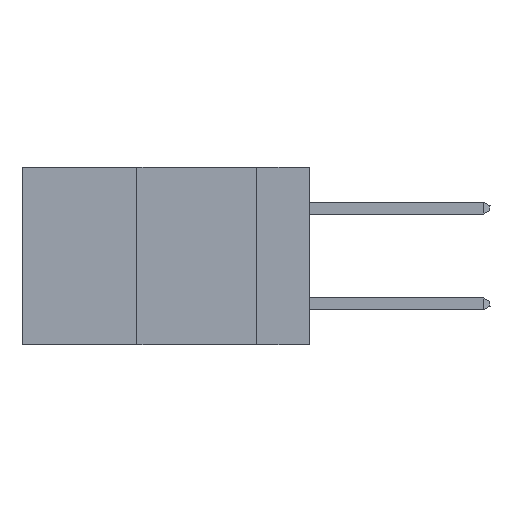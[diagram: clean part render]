
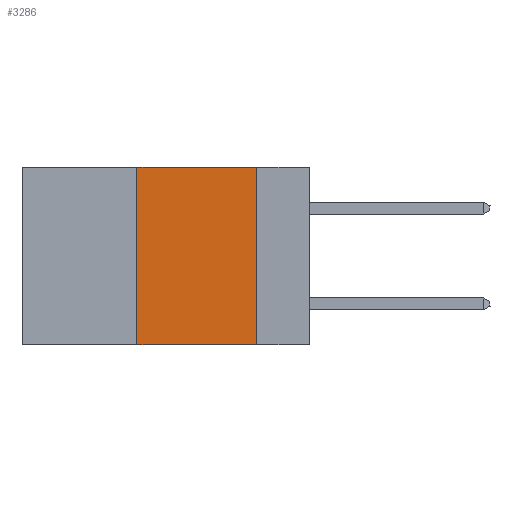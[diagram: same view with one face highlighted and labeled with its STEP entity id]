
A CAD part, left-side view. The second image highlights one B-rep face of the part: STEP entity #3286.
In plain terms, the highlighted planar face has unit normal (-1, 0, 0).
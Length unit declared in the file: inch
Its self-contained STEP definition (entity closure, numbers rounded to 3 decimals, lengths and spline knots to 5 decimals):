
#913 = ORIENTED_EDGE ( 'NONE', *, *, #22457, .F. ) ;
#1438 = CARTESIAN_POINT ( 'NONE',  ( 0., 0.11, 0. ) ) ;
#2616 = VECTOR ( 'NONE', #3526, 39.37008 ) ;
#3018 = FACE_OUTER_BOUND ( 'NONE', #5909, .T. ) ;
#3286 = ADVANCED_FACE ( 'NONE', ( #3018 ), #4682, .F. ) ;
#3526 = DIRECTION ( 'NONE',  ( 0., -1., 0. ) ) ;
#4585 = DIRECTION ( 'NONE',  ( 0., 0., -1. ) ) ;
#4609 = DIRECTION ( 'NONE',  ( 1., 0., 0. ) ) ;
#4682 = PLANE ( 'NONE',  #16794 ) ;
#5305 = CARTESIAN_POINT ( 'NONE',  ( 0., 0.6, 0. ) ) ;
#5696 = CARTESIAN_POINT ( 'NONE',  ( 0., 0.6, -0.37 ) ) ;
#5909 = EDGE_LOOP ( 'NONE', ( #913, #21575, #17641, #16185 ) ) ;
#7152 = VECTOR ( 'NONE', #26349, 39.37008 ) ;
#7170 = EDGE_CURVE ( 'NONE', #22825, #26252, #25528, .T. ) ;
#7497 = VECTOR ( 'NONE', #25679, 39.37008 ) ;
#8321 = LINE ( 'NONE', #27254, #19901 ) ;
#10081 = VERTEX_POINT ( 'NONE', #1438 ) ;
#12664 = EDGE_CURVE ( 'NONE', #16886, #10081, #21799, .T. ) ;
#14945 = EDGE_CURVE ( 'NONE', #22825, #16886, #8321, .T. ) ;
#16185 = ORIENTED_EDGE ( 'NONE', *, *, #7170, .T. ) ;
#16794 = AXIS2_PLACEMENT_3D ( 'NONE', #5305, #4609, #4585 ) ;
#16886 = VERTEX_POINT ( 'NONE', #16931 ) ;
#16931 = CARTESIAN_POINT ( 'NONE',  ( 0., 0.36, 0. ) ) ;
#17641 = ORIENTED_EDGE ( 'NONE', *, *, #14945, .F. ) ;
#19901 = VECTOR ( 'NONE', #20473, 39.37008 ) ;
#20084 = CARTESIAN_POINT ( 'NONE',  ( 0., 0.36, -0.37 ) ) ;
#20473 = DIRECTION ( 'NONE',  ( 0., 0., 1. ) ) ;
#21575 = ORIENTED_EDGE ( 'NONE', *, *, #12664, .F. ) ;
#21799 = LINE ( 'NONE', #26336, #2616 ) ;
#22457 = EDGE_CURVE ( 'NONE', #10081, #26252, #25878, .T. ) ;
#22825 = VERTEX_POINT ( 'NONE', #20084 ) ;
#23389 = CARTESIAN_POINT ( 'NONE',  ( 0., 0.11, 0. ) ) ;
#25528 = LINE ( 'NONE', #5696, #7152 ) ;
#25679 = DIRECTION ( 'NONE',  ( 0., 0., -1. ) ) ;
#25878 = LINE ( 'NONE', #23389, #7497 ) ;
#26252 = VERTEX_POINT ( 'NONE', #29306 ) ;
#26336 = CARTESIAN_POINT ( 'NONE',  ( 0., 0.6, 0. ) ) ;
#26349 = DIRECTION ( 'NONE',  ( 0., -1., 0. ) ) ;
#27254 = CARTESIAN_POINT ( 'NONE',  ( 0., 0.36, 0. ) ) ;
#29306 = CARTESIAN_POINT ( 'NONE',  ( 0., 0.11, -0.37 ) ) ;
